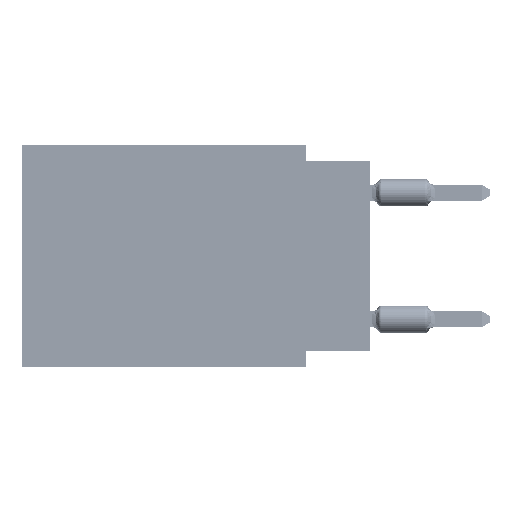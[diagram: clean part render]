
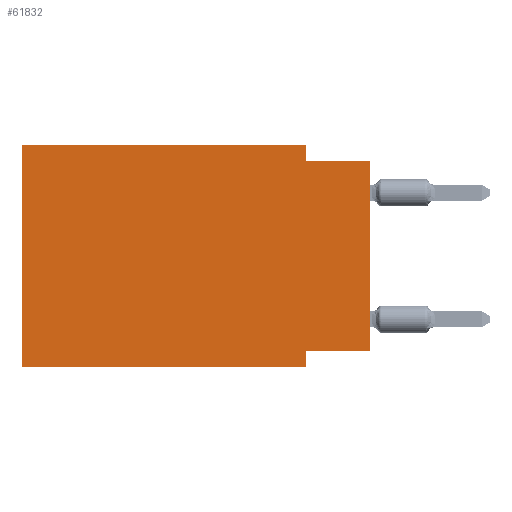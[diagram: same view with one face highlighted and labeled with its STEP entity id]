
A CAD part, left-side view. The second image highlights one B-rep face of the part: STEP entity #61832.
In plain terms, the highlighted planar face has unit normal (-1, 0, 0).
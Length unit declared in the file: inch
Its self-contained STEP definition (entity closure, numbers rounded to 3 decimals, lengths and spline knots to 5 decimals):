
#1093 = CARTESIAN_POINT ( 'NONE',  ( 0., 0.1, 0. ) ) ;
#1315 = CARTESIAN_POINT ( 'NONE',  ( 0., 0.1, 0. ) ) ;
#1650 = ORIENTED_EDGE ( 'NONE', *, *, #44244, .F. ) ;
#5887 = VECTOR ( 'NONE', #48588, 39.37008 ) ;
#6477 = LINE ( 'NONE', #83331, #5887 ) ;
#8670 = CARTESIAN_POINT ( 'NONE',  ( 0., 0.55, 0. ) ) ;
#10924 = CARTESIAN_POINT ( 'NONE',  ( 0., 0., -0.325 ) ) ;
#14703 = LINE ( 'NONE', #48940, #46307 ) ;
#14752 = VERTEX_POINT ( 'NONE', #22072 ) ;
#16277 = LINE ( 'NONE', #1093, #70681 ) ;
#18245 = EDGE_LOOP ( 'NONE', ( #62541, #47462, #75015, #93046, #27645, #49001, #1650, #57358 ) ) ;
#22072 = CARTESIAN_POINT ( 'NONE',  ( 0., 0.1, -0.325 ) ) ;
#22691 = EDGE_CURVE ( 'NONE', #99524, #46144, #61574, .T. ) ;
#26688 = CARTESIAN_POINT ( 'NONE',  ( 0., 0.55, 0. ) ) ;
#27645 = ORIENTED_EDGE ( 'NONE', *, *, #100331, .F. ) ;
#34012 = PLANE ( 'NONE',  #105183 ) ;
#41588 = CARTESIAN_POINT ( 'NONE',  ( 0., 0.55, 0. ) ) ;
#43871 = EDGE_CURVE ( 'NONE', #93671, #83258, #84187, .T. ) ;
#44244 = EDGE_CURVE ( 'NONE', #14752, #62022, #101434, .T. ) ;
#44306 = DIRECTION ( 'NONE',  ( 0., 0., -1. ) ) ;
#44518 = CARTESIAN_POINT ( 'NONE',  ( 0., 0., -0.325 ) ) ;
#45743 = CARTESIAN_POINT ( 'NONE',  ( 0., 0., -0.025 ) ) ;
#46144 = VERTEX_POINT ( 'NONE', #45743 ) ;
#46307 = VECTOR ( 'NONE', #73057, 39.37008 ) ;
#47371 = VECTOR ( 'NONE', #92045, 39.37008 ) ;
#47462 = ORIENTED_EDGE ( 'NONE', *, *, #80808, .F. ) ;
#48588 = DIRECTION ( 'NONE',  ( 0., -1., 0. ) ) ;
#48940 = CARTESIAN_POINT ( 'NONE',  ( 0., 0.55, -0.35 ) ) ;
#49001 = ORIENTED_EDGE ( 'NONE', *, *, #102138, .T. ) ;
#52668 = CARTESIAN_POINT ( 'NONE',  ( 0., 0.55, 0. ) ) ;
#54693 = LINE ( 'NONE', #10924, #106889 ) ;
#56034 = CARTESIAN_POINT ( 'NONE',  ( 0., 0.1, -0.025 ) ) ;
#56073 = DIRECTION ( 'NONE',  ( 0., 0., -1. ) ) ;
#57358 = ORIENTED_EDGE ( 'NONE', *, *, #60834, .F. ) ;
#57727 = CARTESIAN_POINT ( 'NONE',  ( 0., 0.1, -0.35 ) ) ;
#58652 = EDGE_CURVE ( 'NONE', #83258, #73182, #16277, .T. ) ;
#60530 = LINE ( 'NONE', #52668, #110426 ) ;
#60834 = EDGE_CURVE ( 'NONE', #99524, #14752, #54693, .T. ) ;
#61574 = LINE ( 'NONE', #94113, #77338 ) ;
#61832 = ADVANCED_FACE ( 'NONE', ( #76621 ), #34012, .F. ) ;
#62022 = VERTEX_POINT ( 'NONE', #88341 ) ;
#62541 = ORIENTED_EDGE ( 'NONE', *, *, #22691, .T. ) ;
#68219 = DIRECTION ( 'NONE',  ( 1., 0., 0. ) ) ;
#70060 = CARTESIAN_POINT ( 'NONE',  ( 0., 0.55, -0.35 ) ) ;
#70681 = VECTOR ( 'NONE', #44306, 39.37008 ) ;
#71878 = VERTEX_POINT ( 'NONE', #70060 ) ;
#73057 = DIRECTION ( 'NONE',  ( 0., -1., 0. ) ) ;
#73182 = VERTEX_POINT ( 'NONE', #56034 ) ;
#75015 = ORIENTED_EDGE ( 'NONE', *, *, #58652, .F. ) ;
#76621 = FACE_OUTER_BOUND ( 'NONE', #18245, .T. ) ;
#77338 = VECTOR ( 'NONE', #96312, 39.37008 ) ;
#80808 = EDGE_CURVE ( 'NONE', #73182, #46144, #6477, .T. ) ;
#83258 = VERTEX_POINT ( 'NONE', #1315 ) ;
#83331 = CARTESIAN_POINT ( 'NONE',  ( 0., 0., -0.025 ) ) ;
#84187 = LINE ( 'NONE', #41588, #47371 ) ;
#88341 = CARTESIAN_POINT ( 'NONE',  ( 0., 0.1, -0.35 ) ) ;
#88879 = DIRECTION ( 'NONE',  ( 0., 1., 0. ) ) ;
#92045 = DIRECTION ( 'NONE',  ( 0., -1., 0. ) ) ;
#93046 = ORIENTED_EDGE ( 'NONE', *, *, #43871, .F. ) ;
#93671 = VERTEX_POINT ( 'NONE', #8670 ) ;
#94113 = CARTESIAN_POINT ( 'NONE',  ( 0., 0., 0. ) ) ;
#94731 = DIRECTION ( 'NONE',  ( 0., 0., 1. ) ) ;
#96312 = DIRECTION ( 'NONE',  ( 0., 0., 1. ) ) ;
#99524 = VERTEX_POINT ( 'NONE', #44518 ) ;
#100331 = EDGE_CURVE ( 'NONE', #71878, #93671, #60530, .T. ) ;
#101434 = LINE ( 'NONE', #57727, #106553 ) ;
#102138 = EDGE_CURVE ( 'NONE', #71878, #62022, #14703, .T. ) ;
#102437 = DIRECTION ( 'NONE',  ( 0., 0., -1. ) ) ;
#105183 = AXIS2_PLACEMENT_3D ( 'NONE', #26688, #68219, #102437 ) ;
#106553 = VECTOR ( 'NONE', #56073, 39.37008 ) ;
#106889 = VECTOR ( 'NONE', #88879, 39.37008 ) ;
#110426 = VECTOR ( 'NONE', #94731, 39.37008 ) ;
